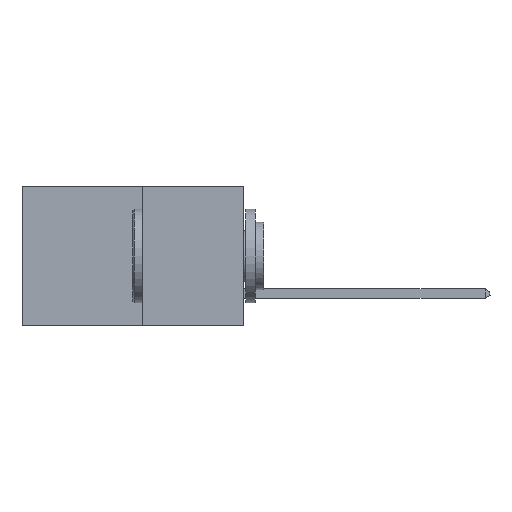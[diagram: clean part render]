
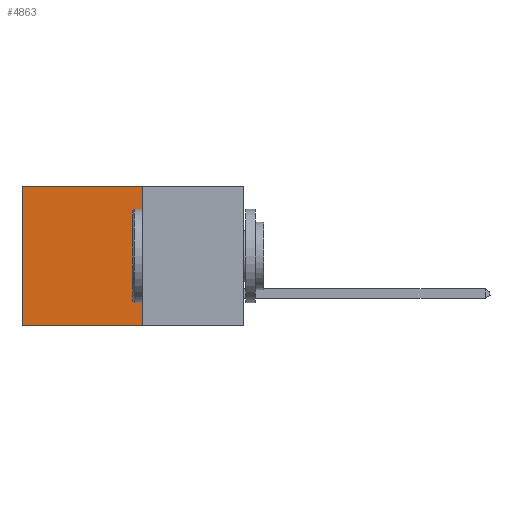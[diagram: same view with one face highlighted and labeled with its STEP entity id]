
A CAD part, left-side view. The second image highlights one B-rep face of the part: STEP entity #4863.
In plain terms, the highlighted planar face has unit normal (-1, 0, 0).
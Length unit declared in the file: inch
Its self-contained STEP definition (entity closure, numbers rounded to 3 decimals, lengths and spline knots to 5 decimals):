
#409 = CARTESIAN_POINT ( 'NONE',  ( 0.277, 0.27, -0.37 ) ) ;
#825 = EDGE_CURVE ( 'NONE', #3162, #3704, #11025, .T. ) ;
#911 = LINE ( 'NONE', #4631, #1184 ) ;
#1184 = VECTOR ( 'NONE', #1935, 39.37008 ) ;
#1286 = DIRECTION ( 'NONE',  ( 0., 0., -1. ) ) ;
#1935 = DIRECTION ( 'NONE',  ( 0., 1., 0. ) ) ;
#2371 = AXIS2_PLACEMENT_3D ( 'NONE', #4507, #4471, #4468 ) ;
#2778 = VECTOR ( 'NONE', #1286, 39.37008 ) ;
#2901 = CARTESIAN_POINT ( 'NONE',  ( 0.277, 0.59, -0.37 ) ) ;
#3111 = EDGE_LOOP ( 'NONE', ( #8226, #8316, #5103, #4666 ) ) ;
#3144 = EDGE_CURVE ( 'NONE', #3162, #9127, #5197, .T. ) ;
#3162 = VERTEX_POINT ( 'NONE', #7975 ) ;
#3580 = LINE ( 'NONE', #2901, #7658 ) ;
#3704 = VERTEX_POINT ( 'NONE', #3764 ) ;
#3764 = CARTESIAN_POINT ( 'NONE',  ( 0.277, 0.59, 0. ) ) ;
#4468 = DIRECTION ( 'NONE',  ( 0., 0., -1. ) ) ;
#4471 = DIRECTION ( 'NONE',  ( 1., 0., 0. ) ) ;
#4496 = PLANE ( 'NONE',  #2371 ) ;
#4507 = CARTESIAN_POINT ( 'NONE',  ( 0.277, 0.27, -0.37 ) ) ;
#4631 = CARTESIAN_POINT ( 'NONE',  ( 0.277, 0.27, -0.37 ) ) ;
#4666 = ORIENTED_EDGE ( 'NONE', *, *, #825, .T. ) ;
#4863 = ADVANCED_FACE ( 'NONE', ( #6300 ), #4496, .F. ) ;
#5103 = ORIENTED_EDGE ( 'NONE', *, *, #3144, .F. ) ;
#5197 = LINE ( 'NONE', #5789, #2778 ) ;
#5789 = CARTESIAN_POINT ( 'NONE',  ( 0.277, 0.27, -0.37 ) ) ;
#6300 = FACE_OUTER_BOUND ( 'NONE', #3111, .T. ) ;
#6678 = VECTOR ( 'NONE', #9826, 39.37008 ) ;
#7517 = VERTEX_POINT ( 'NONE', #8772 ) ;
#7658 = VECTOR ( 'NONE', #8886, 39.37008 ) ;
#7975 = CARTESIAN_POINT ( 'NONE',  ( 0.277, 0.27, 0. ) ) ;
#8188 = EDGE_CURVE ( 'NONE', #3704, #7517, #3580, .T. ) ;
#8226 = ORIENTED_EDGE ( 'NONE', *, *, #8188, .T. ) ;
#8316 = ORIENTED_EDGE ( 'NONE', *, *, #9519, .F. ) ;
#8772 = CARTESIAN_POINT ( 'NONE',  ( 0.277, 0.59, -0.37 ) ) ;
#8886 = DIRECTION ( 'NONE',  ( 0., 0., -1. ) ) ;
#9127 = VERTEX_POINT ( 'NONE', #409 ) ;
#9232 = CARTESIAN_POINT ( 'NONE',  ( 0.277, 0.27, 0. ) ) ;
#9519 = EDGE_CURVE ( 'NONE', #9127, #7517, #911, .T. ) ;
#9826 = DIRECTION ( 'NONE',  ( 0., 1., 0. ) ) ;
#11025 = LINE ( 'NONE', #9232, #6678 ) ;
